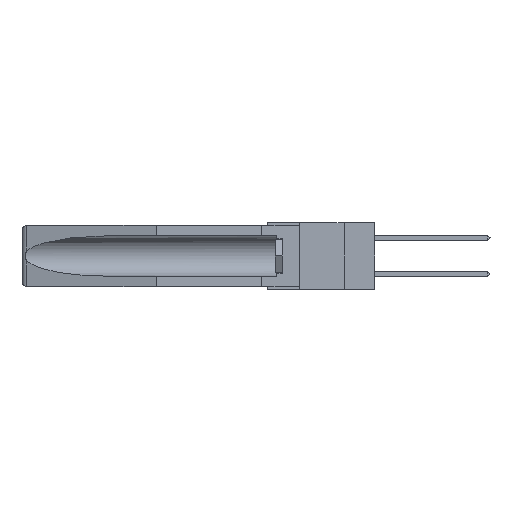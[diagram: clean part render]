
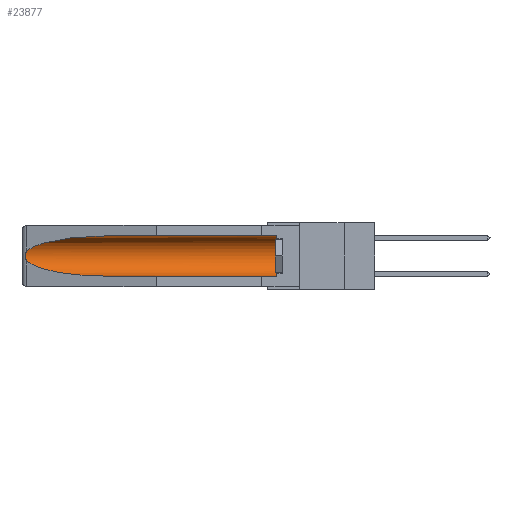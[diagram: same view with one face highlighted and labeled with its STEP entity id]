
A CAD part, left-side view. The second image highlights one B-rep face of the part: STEP entity #23877.
In plain terms, the highlighted cylindrical face has radius 2.857 mm (diameter 5.715 mm), a partial arc.
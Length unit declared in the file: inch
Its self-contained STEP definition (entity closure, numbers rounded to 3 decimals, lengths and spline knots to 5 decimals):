
#67 = VERTEX_POINT ( 'NONE', #15561 ) ;
#492 = VECTOR ( 'NONE', #22047, 39.37008 ) ;
#615 = CARTESIAN_POINT ( 'NONE',  ( 0.155, 1.07973, -0.284 ) ) ;
#1375 = CARTESIAN_POINT ( 'NONE',  ( 0.25451, 1.48313, -0.24835 ) ) ;
#1653 = DIRECTION ( 'NONE',  ( 0., 0., 1. ) ) ;
#1724 = CARTESIAN_POINT ( 'NONE',  ( 0.155, 1.07973, -0.059 ) ) ;
#1977 = CARTESIAN_POINT ( 'NONE',  ( 0.155, 1.07973, -0.059 ) ) ;
#2261 = CIRCLE ( 'NONE', #20670, 0.1125 ) ;
#2379 = EDGE_CURVE ( 'NONE', #14406, #11640, #19604, .T. ) ;
#2705 = ORIENTED_EDGE ( 'NONE', *, *, #2379, .T. ) ;
#2822 = ORIENTED_EDGE ( 'NONE', *, *, #7478, .T. ) ;
#3426 = CARTESIAN_POINT ( 'NONE',  ( 0.26655, 1.53094, -0.18657 ) ) ;
#3744 = CARTESIAN_POINT ( 'NONE',  ( 0.155, 1.07973, -0.284 ) ) ;
#3837 = DIRECTION ( 'NONE',  ( 0., 1., 0. ) ) ;
#5407 = CARTESIAN_POINT ( 'NONE',  ( 0.155, 0.126, -0.1715 ) ) ;
#5589 = DIRECTION ( 'NONE',  ( 0., 0., 1. ) ) ;
#5724 = EDGE_CURVE ( 'NONE', #11640, #25182, #17950, .T. ) ;
#5851 = DIRECTION ( 'NONE',  ( 0., 1., 0. ) ) ;
#5908 = CARTESIAN_POINT ( 'NONE',  ( 0.21114, 1.30732, -0.059 ) ) ;
#6000 = CARTESIAN_POINT ( 'NONE',  ( 0.25451, 1.48313, -0.09465 ) ) ;
#7420 = CARTESIAN_POINT ( 'NONE',  ( 0.2673, 1.5327, -0.16383 ) ) ;
#7478 = EDGE_CURVE ( 'NONE', #21963, #67, #2261, .T. ) ;
#7500 = AXIS2_PLACEMENT_3D ( 'NONE', #16215, #3837, #1653 ) ;
#7691 = CARTESIAN_POINT ( 'NONE',  ( 0.2673, 1.53269, -0.17917 ) ) ;
#7748 = CARTESIAN_POINT ( 'NONE',  ( 0.21114, 1.30732, -0.284 ) ) ;
#7782 = CARTESIAN_POINT ( 'NONE',  ( 0.26597, 1.52961, -0.15275 ) ) ;
#9567 = ORIENTED_EDGE ( 'NONE', *, *, #9990, .F. ) ;
#9608 = CARTESIAN_POINT ( 'NONE',  ( 0.26537, 1.52718, -0.19328 ) ) ;
#9857 = CARTESIAN_POINT ( 'NONE',  ( 0.2675, 1.53308, -0.17534 ) ) ;
#9990 = EDGE_CURVE ( 'NONE', #21963, #25182, #14783, .T. ) ;
#10541 = VERTEX_POINT ( 'NONE', #1977 ) ;
#10931 = FACE_OUTER_BOUND ( 'NONE', #15335, .T. ) ;
#11307 = CARTESIAN_POINT ( 'NONE',  ( 0.26537, 1.52718, -0.19328 ) ) ;
#11640 = VERTEX_POINT ( 'NONE', #11307 ) ;
#11898 = CARTESIAN_POINT ( 'NONE',  ( 0.155, -0.30754, -0.284 ) ) ;
#12031 = ORIENTED_EDGE ( 'NONE', *, *, #5724, .T. ) ;
#12859 = ORIENTED_EDGE ( 'NONE', *, *, #19977, .T. ) ;
#13790 = CARTESIAN_POINT ( 'NONE',  ( 0.26537, 1.52718, -0.19328 ) ) ;
#14074 = LINE ( 'NONE', #26087, #15649 ) ;
#14395 = CARTESIAN_POINT ( 'NONE',  ( 0.26537, 1.52718, -0.14972 ) ) ;
#14406 = VERTEX_POINT ( 'NONE', #24258 ) ;
#14783 = LINE ( 'NONE', #11898, #492 ) ;
#15188 =( BOUNDED_CURVE ( )  B_SPLINE_CURVE ( 3, ( #1724, #5908, #6000, #14395 ),
 .UNSPECIFIED., .F., .T. ) 
 B_SPLINE_CURVE_WITH_KNOTS ( ( 4, 4 ),
 ( 4.71239, 6.08839 ),
 .UNSPECIFIED. ) 
 CURVE ( )  GEOMETRIC_REPRESENTATION_ITEM ( )  RATIONAL_B_SPLINE_CURVE ( ( 1., 0.848, 0.848, 1. ) ) 
 REPRESENTATION_ITEM ( '' )  );
#15335 = EDGE_LOOP ( 'NONE', ( #20191, #2705, #12031, #9567, #2822, #12859 ) ) ;
#15561 = CARTESIAN_POINT ( 'NONE',  ( 0.155, 0.126, -0.059 ) ) ;
#15649 = VECTOR ( 'NONE', #5851, 39.37008 ) ;
#15975 = CARTESIAN_POINT ( 'NONE',  ( 0.26597, 1.5296, -0.19026 ) ) ;
#16215 = CARTESIAN_POINT ( 'NONE',  ( 0.155, -0.30754, -0.1715 ) ) ;
#17682 = CARTESIAN_POINT ( 'NONE',  ( 0.2675, 1.53308, -0.16763 ) ) ;
#17925 = CARTESIAN_POINT ( 'NONE',  ( 0.26654, 1.53092, -0.15636 ) ) ;
#17950 =( BOUNDED_CURVE ( )  B_SPLINE_CURVE ( 3, ( #13790, #1375, #7748, #3744 ),
 .UNSPECIFIED., .F., .F. ) 
 B_SPLINE_CURVE_WITH_KNOTS ( ( 4, 4 ),
 ( 0.1948, 1.5708 ),
 .UNSPECIFIED. ) 
 CURVE ( )  GEOMETRIC_REPRESENTATION_ITEM ( )  RATIONAL_B_SPLINE_CURVE ( ( 1., 0.848, 0.848, 1. ) ) 
 REPRESENTATION_ITEM ( '' )  );
#18201 = EDGE_CURVE ( 'NONE', #10541, #14406, #15188, .T. ) ;
#19604 = B_SPLINE_CURVE_WITH_KNOTS ( 'NONE', 3,
 ( #26195, #7782, #17925, #7420, #17682, #9857, #7691, #3426, #15975, #9608 ),
 .UNSPECIFIED., .F., .F.,
 ( 4, 2, 2, 2, 4 ),
 ( 0., 0.00029, 0.00058, 0.00087, 0.00117 ),
 .UNSPECIFIED. ) ;
#19977 = EDGE_CURVE ( 'NONE', #67, #10541, #14074, .T. ) ;
#20191 = ORIENTED_EDGE ( 'NONE', *, *, #18201, .T. ) ;
#20670 = AXIS2_PLACEMENT_3D ( 'NONE', #5407, #21681, #5589 ) ;
#21681 = DIRECTION ( 'NONE',  ( 0., -1., 0. ) ) ;
#21963 = VERTEX_POINT ( 'NONE', #23477 ) ;
#22047 = DIRECTION ( 'NONE',  ( 0., 1., 0. ) ) ;
#23477 = CARTESIAN_POINT ( 'NONE',  ( 0.155, 0.126, -0.284 ) ) ;
#23877 = ADVANCED_FACE ( 'NONE', ( #10931 ), #26722, .F. ) ;
#24258 = CARTESIAN_POINT ( 'NONE',  ( 0.26537, 1.52718, -0.14972 ) ) ;
#25182 = VERTEX_POINT ( 'NONE', #615 ) ;
#26087 = CARTESIAN_POINT ( 'NONE',  ( 0.155, -0.30754, -0.059 ) ) ;
#26195 = CARTESIAN_POINT ( 'NONE',  ( 0.26537, 1.52718, -0.14972 ) ) ;
#26722 = CYLINDRICAL_SURFACE ( 'NONE', #7500, 0.1125 ) ;
